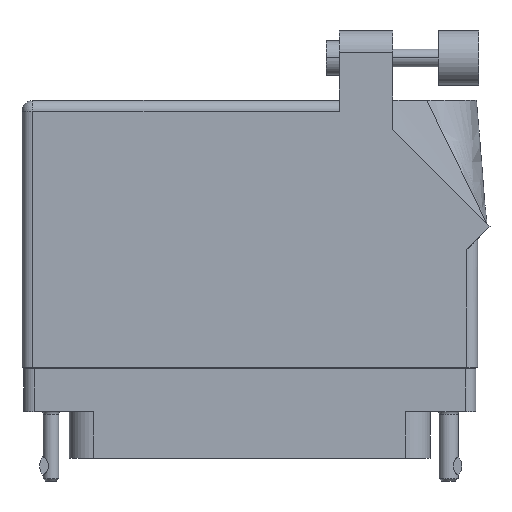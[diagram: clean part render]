
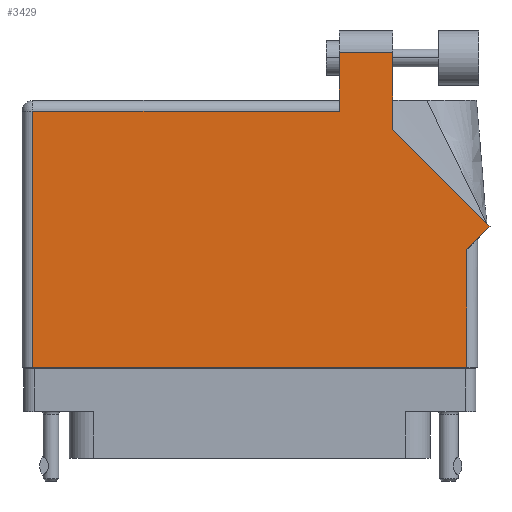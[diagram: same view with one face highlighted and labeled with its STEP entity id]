
A CAD part, front view. The second image highlights one B-rep face of the part: STEP entity #3429.
In plain terms, the highlighted face is planar.
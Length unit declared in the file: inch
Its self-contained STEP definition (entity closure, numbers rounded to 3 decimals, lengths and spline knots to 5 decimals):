
#1058 = DIRECTION ( 'NONE',  ( -0.707, 0.707, 0. ) ) ;
#2131 = ORIENTED_EDGE ( 'NONE', *, *, #11358, .T. ) ;
#3429 = ADVANCED_FACE ( 'NONE', ( #42513 ), #32916, .F. ) ;
#3479 = LINE ( 'NONE', #45343, #56637 ) ;
#3526 = EDGE_LOOP ( 'NONE', ( #27704, #2131, #34304, #40954, #26512, #31480, #55459, #41112, #55279 ) ) ;
#4448 = DIRECTION ( 'NONE',  ( 0., 0., -1. ) ) ;
#5158 = CARTESIAN_POINT ( 'NONE',  ( -1.306, 1.368, 0.455 ) ) ;
#5247 = DIRECTION ( 'NONE',  ( 1., 0., 0. ) ) ;
#7286 = VERTEX_POINT ( 'NONE', #9075 ) ;
#8200 = LINE ( 'NONE', #38292, #18528 ) ;
#8712 = CARTESIAN_POINT ( 'NONE',  ( -1.244, -0.1, 0.455 ) ) ;
#9075 = CARTESIAN_POINT ( 'NONE',  ( -1.244, 1.368, 0.455 ) ) ;
#11358 = EDGE_CURVE ( 'NONE', #53808, #19186, #15896, .T. ) ;
#15712 = VERTEX_POINT ( 'NONE', #50531 ) ;
#15896 = LINE ( 'NONE', #35039, #42577 ) ;
#16347 = CARTESIAN_POINT ( 'NONE',  ( 0.513, 1.43, 0.455 ) ) ;
#16675 = DIRECTION ( 'NONE',  ( 0., 1., 0. ) ) ;
#17039 = CARTESIAN_POINT ( 'NONE',  ( 0.82, 1.705, 0.455 ) ) ;
#17421 = DIRECTION ( 'NONE',  ( 0., -1., 0. ) ) ;
#18528 = VECTOR ( 'NONE', #5247, 39.37008 ) ;
#18849 = CARTESIAN_POINT ( 'NONE',  ( 1.306, 0.637, 0.455 ) ) ;
#19186 = VERTEX_POINT ( 'NONE', #45768 ) ;
#19967 = CARTESIAN_POINT ( 'NONE',  ( 1.244, 0.575, 0.455 ) ) ;
#20567 = VERTEX_POINT ( 'NONE', #19967 ) ;
#20805 = DIRECTION ( 'NONE',  ( -1., 0., 0. ) ) ;
#20894 = DIRECTION ( 'NONE',  ( 0., -1., 0. ) ) ;
#22963 = VECTOR ( 'NONE', #16675, 39.37008 ) ;
#23104 = LINE ( 'NONE', #8712, #59987 ) ;
#23301 = LINE ( 'NONE', #18849, #34355 ) ;
#23418 = CARTESIAN_POINT ( 'NONE',  ( -1.306, 1.43, 0.455 ) ) ;
#25570 = EDGE_CURVE ( 'NONE', #44246, #20567, #46702, .T. ) ;
#26512 = ORIENTED_EDGE ( 'NONE', *, *, #28686, .T. ) ;
#27704 = ORIENTED_EDGE ( 'NONE', *, *, #43696, .T. ) ;
#28485 = VERTEX_POINT ( 'NONE', #30370 ) ;
#28686 = EDGE_CURVE ( 'NONE', #7286, #45447, #23104, .T. ) ;
#30370 = CARTESIAN_POINT ( 'NONE',  ( 0.82, 1.26442, 0.455 ) ) ;
#31480 = ORIENTED_EDGE ( 'NONE', *, *, #37023, .T. ) ;
#32300 = LINE ( 'NONE', #39509, #46441 ) ;
#32916 = PLANE ( 'NONE',  #37393 ) ;
#33038 = DIRECTION ( 'NONE',  ( 0.707, 0.707, 0. ) ) ;
#33100 = DIRECTION ( 'NONE',  ( -1., 0., 0. ) ) ;
#33226 = CARTESIAN_POINT ( 'NONE',  ( 1.244, -0.1, 0.455 ) ) ;
#34304 = ORIENTED_EDGE ( 'NONE', *, *, #45413, .T. ) ;
#34355 = VECTOR ( 'NONE', #33038, 39.37008 ) ;
#34805 = EDGE_CURVE ( 'NONE', #38412, #7286, #60129, .T. ) ;
#34905 = CARTESIAN_POINT ( 'NONE',  ( -1.244, -0.1, 0.455 ) ) ;
#35039 = CARTESIAN_POINT ( 'NONE',  ( 0.513, 1.705, 0.455 ) ) ;
#36180 = DIRECTION ( 'NONE',  ( 0., 1., 0. ) ) ;
#37023 = EDGE_CURVE ( 'NONE', #45447, #44246, #8200, .T. ) ;
#37393 = AXIS2_PLACEMENT_3D ( 'NONE', #23418, #4448, #33100 ) ;
#38292 = CARTESIAN_POINT ( 'NONE',  ( -1.306, -0.1, 0.455 ) ) ;
#38412 = VERTEX_POINT ( 'NONE', #60561 ) ;
#38772 = VECTOR ( 'NONE', #20894, 39.37008 ) ;
#38831 = VECTOR ( 'NONE', #57326, 39.37008 ) ;
#39445 = EDGE_CURVE ( 'NONE', #15712, #28485, #32300, .T. ) ;
#39509 = CARTESIAN_POINT ( 'NONE',  ( 1.37671, 0.70771, 0.455 ) ) ;
#40234 = CARTESIAN_POINT ( 'NONE',  ( 1.244, 0.637, 0.455 ) ) ;
#40954 = ORIENTED_EDGE ( 'NONE', *, *, #34805, .T. ) ;
#41112 = ORIENTED_EDGE ( 'NONE', *, *, #44348, .T. ) ;
#42513 = FACE_OUTER_BOUND ( 'NONE', #3526, .T. ) ;
#42577 = VECTOR ( 'NONE', #20805, 39.37008 ) ;
#43696 = EDGE_CURVE ( 'NONE', #28485, #53808, #3479, .T. ) ;
#44246 = VERTEX_POINT ( 'NONE', #33226 ) ;
#44348 = EDGE_CURVE ( 'NONE', #20567, #15712, #23301, .T. ) ;
#45343 = CARTESIAN_POINT ( 'NONE',  ( 0.82, 1.26442, 0.455 ) ) ;
#45413 = EDGE_CURVE ( 'NONE', #19186, #38412, #51380, .T. ) ;
#45447 = VERTEX_POINT ( 'NONE', #34905 ) ;
#45768 = CARTESIAN_POINT ( 'NONE',  ( 0.513, 1.705, 0.455 ) ) ;
#46441 = VECTOR ( 'NONE', #1058, 39.37008 ) ;
#46702 = LINE ( 'NONE', #40234, #22963 ) ;
#50531 = CARTESIAN_POINT ( 'NONE',  ( 1.37671, 0.70771, 0.455 ) ) ;
#51380 = LINE ( 'NONE', #16347, #38772 ) ;
#53808 = VERTEX_POINT ( 'NONE', #17039 ) ;
#55279 = ORIENTED_EDGE ( 'NONE', *, *, #39445, .T. ) ;
#55459 = ORIENTED_EDGE ( 'NONE', *, *, #25570, .T. ) ;
#56637 = VECTOR ( 'NONE', #36180, 39.37008 ) ;
#57326 = DIRECTION ( 'NONE',  ( -1., 0., 0. ) ) ;
#59987 = VECTOR ( 'NONE', #17421, 39.37008 ) ;
#60129 = LINE ( 'NONE', #5158, #38831 ) ;
#60561 = CARTESIAN_POINT ( 'NONE',  ( 0.513, 1.368, 0.455 ) ) ;
